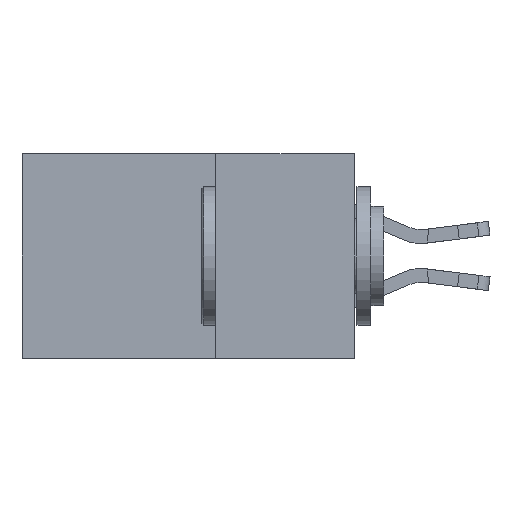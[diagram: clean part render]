
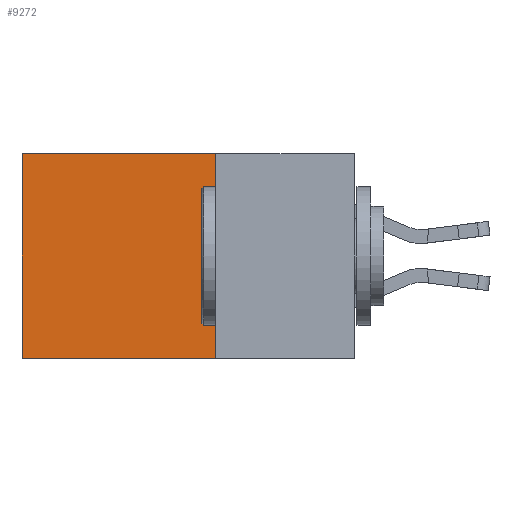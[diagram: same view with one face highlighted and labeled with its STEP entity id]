
A CAD part, left-side view. The second image highlights one B-rep face of the part: STEP entity #9272.
In plain terms, the highlighted planar face has unit normal (-1, 0, 0).
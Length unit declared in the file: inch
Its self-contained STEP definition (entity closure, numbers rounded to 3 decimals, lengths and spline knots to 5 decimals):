
#31 = LINE ( 'NONE', #11087, #5678 ) ;
#526 = DIRECTION ( 'NONE',  ( 0., 0., -1. ) ) ;
#1126 = LINE ( 'NONE', #7110, #12181 ) ;
#1615 = ORIENTED_EDGE ( 'NONE', *, *, #2898, .T. ) ;
#2264 = EDGE_CURVE ( 'NONE', #11925, #9599, #31, .T. ) ;
#2791 = VECTOR ( 'NONE', #526, 39.37008 ) ;
#2898 = EDGE_CURVE ( 'NONE', #9599, #14415, #1126, .T. ) ;
#3436 = EDGE_CURVE ( 'NONE', #11925, #15119, #15480, .T. ) ;
#3710 = CARTESIAN_POINT ( 'NONE',  ( 0.298, 0.25, 0. ) ) ;
#3768 = PLANE ( 'NONE',  #14167 ) ;
#3794 = ORIENTED_EDGE ( 'NONE', *, *, #8098, .F. ) ;
#4007 = VECTOR ( 'NONE', #9806, 39.37008 ) ;
#5148 = DIRECTION ( 'NONE',  ( 0., 1., 0. ) ) ;
#5678 = VECTOR ( 'NONE', #5148, 39.37008 ) ;
#5715 = ORIENTED_EDGE ( 'NONE', *, *, #3436, .F. ) ;
#6191 = DIRECTION ( 'NONE',  ( 1., 0., 0. ) ) ;
#7110 = CARTESIAN_POINT ( 'NONE',  ( 0.298, 0.6, 0. ) ) ;
#7932 = LINE ( 'NONE', #12211, #4007 ) ;
#8060 = CARTESIAN_POINT ( 'NONE',  ( 0.298, 0.25, -0.37 ) ) ;
#8098 = EDGE_CURVE ( 'NONE', #15119, #14415, #7932, .T. ) ;
#8358 = DIRECTION ( 'NONE',  ( 0., 0., -1. ) ) ;
#8375 = DIRECTION ( 'NONE',  ( 0., 0., -1. ) ) ;
#9272 = ADVANCED_FACE ( 'NONE', ( #12705 ), #3768, .F. ) ;
#9394 = CARTESIAN_POINT ( 'NONE',  ( 0.298, 0.25, 0. ) ) ;
#9599 = VERTEX_POINT ( 'NONE', #14087 ) ;
#9806 = DIRECTION ( 'NONE',  ( 0., 1., 0. ) ) ;
#10000 = CARTESIAN_POINT ( 'NONE',  ( 0.298, 0.25, 0. ) ) ;
#11087 = CARTESIAN_POINT ( 'NONE',  ( 0.298, 0.25, 0. ) ) ;
#11646 = CARTESIAN_POINT ( 'NONE',  ( 0.298, 0.6, -0.37 ) ) ;
#11925 = VERTEX_POINT ( 'NONE', #9394 ) ;
#12181 = VECTOR ( 'NONE', #8358, 39.37008 ) ;
#12211 = CARTESIAN_POINT ( 'NONE',  ( 0.298, 0.25, -0.37 ) ) ;
#12705 = FACE_OUTER_BOUND ( 'NONE', #14816, .T. ) ;
#14087 = CARTESIAN_POINT ( 'NONE',  ( 0.298, 0.6, 0. ) ) ;
#14167 = AXIS2_PLACEMENT_3D ( 'NONE', #3710, #6191, #8375 ) ;
#14415 = VERTEX_POINT ( 'NONE', #11646 ) ;
#14509 = ORIENTED_EDGE ( 'NONE', *, *, #2264, .T. ) ;
#14816 = EDGE_LOOP ( 'NONE', ( #1615, #3794, #5715, #14509 ) ) ;
#15119 = VERTEX_POINT ( 'NONE', #8060 ) ;
#15480 = LINE ( 'NONE', #10000, #2791 ) ;
